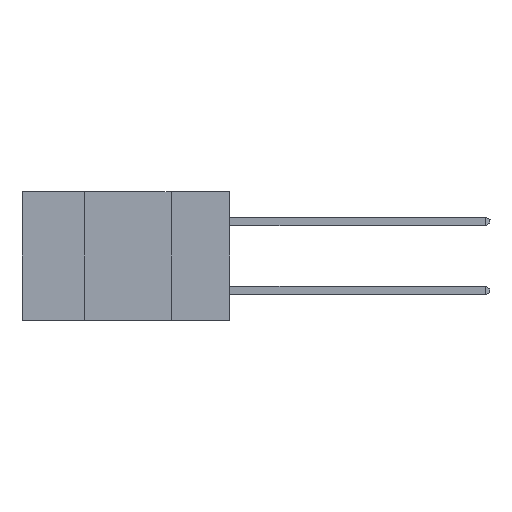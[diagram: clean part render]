
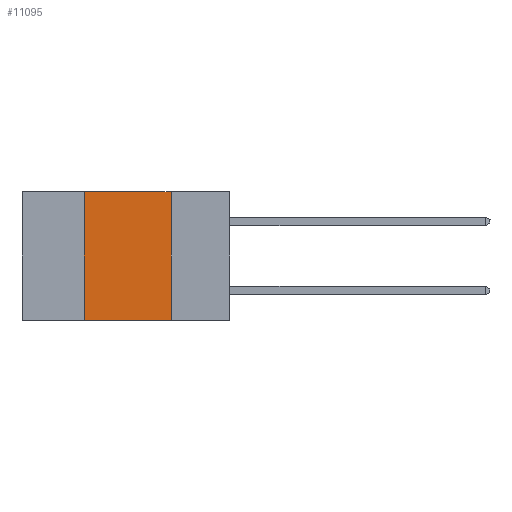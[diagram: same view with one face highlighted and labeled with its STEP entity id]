
A CAD part, left-side view. The second image highlights one B-rep face of the part: STEP entity #11095.
In plain terms, the highlighted planar face has unit normal (-1, 0, 0).
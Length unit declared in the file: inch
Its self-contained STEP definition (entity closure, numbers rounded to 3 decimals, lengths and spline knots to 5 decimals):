
#54 = DIRECTION ( 'NONE',  ( 0., 0., 1. ) ) ;
#296 = VERTEX_POINT ( 'NONE', #15876 ) ;
#298 = VECTOR ( 'NONE', #15109, 39.37008 ) ;
#1364 = DIRECTION ( 'NONE',  ( 0., 0., -1. ) ) ;
#1442 = PLANE ( 'NONE',  #18438 ) ;
#1779 = EDGE_CURVE ( 'NONE', #21570, #3979, #19808, .T. ) ;
#2530 = ORIENTED_EDGE ( 'NONE', *, *, #15365, .F. ) ;
#2908 = LINE ( 'NONE', #18478, #10571 ) ;
#3979 = VERTEX_POINT ( 'NONE', #19679 ) ;
#4878 = DIRECTION ( 'NONE',  ( 0., 0., -1. ) ) ;
#5652 = DIRECTION ( 'NONE',  ( 1., 0., 0. ) ) ;
#6696 = DIRECTION ( 'NONE',  ( 0., -1., 0. ) ) ;
#8047 = CARTESIAN_POINT ( 'NONE',  ( 0., 0.42, 0. ) ) ;
#10571 = VECTOR ( 'NONE', #4878, 39.37008 ) ;
#11095 = ADVANCED_FACE ( 'NONE', ( #13516 ), #1442, .F. ) ;
#11278 = CARTESIAN_POINT ( 'NONE',  ( 0., 0.6, 0. ) ) ;
#11413 = EDGE_CURVE ( 'NONE', #14920, #296, #18370, .T. ) ;
#12179 = VECTOR ( 'NONE', #6696, 39.37008 ) ;
#13516 = FACE_OUTER_BOUND ( 'NONE', #15050, .T. ) ;
#14110 = ORIENTED_EDGE ( 'NONE', *, *, #1779, .T. ) ;
#14920 = VERTEX_POINT ( 'NONE', #8047 ) ;
#15050 = EDGE_LOOP ( 'NONE', ( #20423, #19053, #2530, #14110 ) ) ;
#15109 = DIRECTION ( 'NONE',  ( 0., -1., 0. ) ) ;
#15152 = EDGE_CURVE ( 'NONE', #296, #3979, #2908, .T. ) ;
#15365 = EDGE_CURVE ( 'NONE', #21570, #14920, #18180, .T. ) ;
#15876 = CARTESIAN_POINT ( 'NONE',  ( 0., 0.17, 0. ) ) ;
#17275 = CARTESIAN_POINT ( 'NONE',  ( 0., 0.6, 0. ) ) ;
#18180 = LINE ( 'NONE', #25273, #22123 ) ;
#18370 = LINE ( 'NONE', #11278, #298 ) ;
#18438 = AXIS2_PLACEMENT_3D ( 'NONE', #17275, #5652, #1364 ) ;
#18478 = CARTESIAN_POINT ( 'NONE',  ( 0., 0.17, 0. ) ) ;
#19053 = ORIENTED_EDGE ( 'NONE', *, *, #11413, .F. ) ;
#19679 = CARTESIAN_POINT ( 'NONE',  ( 0., 0.17, -0.37 ) ) ;
#19808 = LINE ( 'NONE', #24873, #12179 ) ;
#20423 = ORIENTED_EDGE ( 'NONE', *, *, #15152, .F. ) ;
#21570 = VERTEX_POINT ( 'NONE', #24339 ) ;
#22123 = VECTOR ( 'NONE', #54, 39.37008 ) ;
#24339 = CARTESIAN_POINT ( 'NONE',  ( 0., 0.42, -0.37 ) ) ;
#24873 = CARTESIAN_POINT ( 'NONE',  ( 0., 0.6, -0.37 ) ) ;
#25273 = CARTESIAN_POINT ( 'NONE',  ( 0., 0.42, 0. ) ) ;
